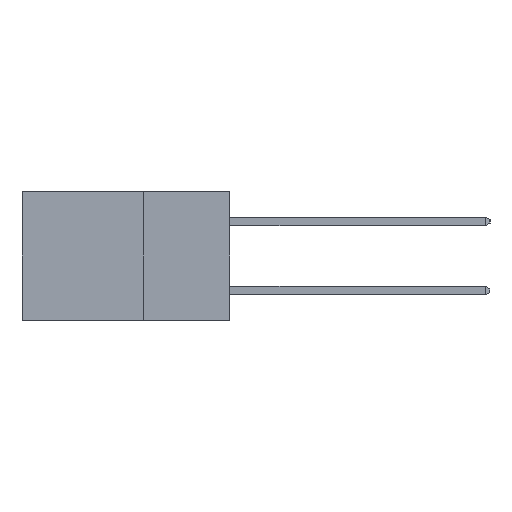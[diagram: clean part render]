
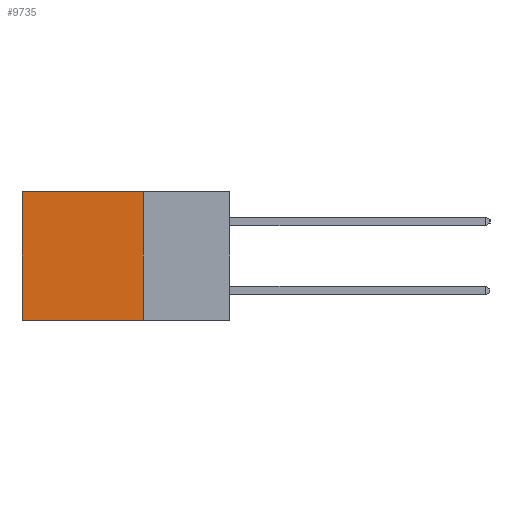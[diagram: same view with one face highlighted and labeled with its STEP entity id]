
A CAD part, left-side view. The second image highlights one B-rep face of the part: STEP entity #9735.
In plain terms, the highlighted planar face has unit normal (-1, 0, 0).
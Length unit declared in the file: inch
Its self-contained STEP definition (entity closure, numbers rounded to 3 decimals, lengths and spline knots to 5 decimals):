
#95 = CARTESIAN_POINT ( 'NONE',  ( 0.298, 0.25, 0. ) ) ;
#1175 = VERTEX_POINT ( 'NONE', #10415 ) ;
#1564 = VERTEX_POINT ( 'NONE', #8498 ) ;
#1645 = DIRECTION ( 'NONE',  ( 0., 1., 0. ) ) ;
#1934 = EDGE_LOOP ( 'NONE', ( #9062, #13494, #11848, #5618 ) ) ;
#1949 = VERTEX_POINT ( 'NONE', #3498 ) ;
#2283 = LINE ( 'NONE', #4247, #5204 ) ;
#2879 = LINE ( 'NONE', #8456, #8440 ) ;
#3411 = LINE ( 'NONE', #8245, #8972 ) ;
#3498 = CARTESIAN_POINT ( 'NONE',  ( 0.298, 0.6, 0. ) ) ;
#3585 = EDGE_CURVE ( 'NONE', #1564, #1949, #2283, .T. ) ;
#4247 = CARTESIAN_POINT ( 'NONE',  ( 0.298, 0.25, 0. ) ) ;
#4409 = FACE_OUTER_BOUND ( 'NONE', #1934, .T. ) ;
#4459 = VERTEX_POINT ( 'NONE', #10061 ) ;
#5204 = VECTOR ( 'NONE', #10838, 39.37008 ) ;
#5450 = VECTOR ( 'NONE', #1645, 39.37008 ) ;
#5618 = ORIENTED_EDGE ( 'NONE', *, *, #3585, .T. ) ;
#5648 = DIRECTION ( 'NONE',  ( 1., 0., 0. ) ) ;
#8245 = CARTESIAN_POINT ( 'NONE',  ( 0.298, 0.6, 0. ) ) ;
#8440 = VECTOR ( 'NONE', #11726, 39.37008 ) ;
#8456 = CARTESIAN_POINT ( 'NONE',  ( 0.298, 0.25, 0. ) ) ;
#8498 = CARTESIAN_POINT ( 'NONE',  ( 0.298, 0.25, 0. ) ) ;
#8774 = LINE ( 'NONE', #13726, #5450 ) ;
#8972 = VECTOR ( 'NONE', #10403, 39.37008 ) ;
#9062 = ORIENTED_EDGE ( 'NONE', *, *, #12751, .T. ) ;
#9312 = EDGE_CURVE ( 'NONE', #1175, #4459, #8774, .T. ) ;
#9735 = ADVANCED_FACE ( 'NONE', ( #4409 ), #10084, .F. ) ;
#10061 = CARTESIAN_POINT ( 'NONE',  ( 0.298, 0.6, -0.37 ) ) ;
#10084 = PLANE ( 'NONE',  #11988 ) ;
#10403 = DIRECTION ( 'NONE',  ( 0., 0., -1. ) ) ;
#10415 = CARTESIAN_POINT ( 'NONE',  ( 0.298, 0.25, -0.37 ) ) ;
#10838 = DIRECTION ( 'NONE',  ( 0., 1., 0. ) ) ;
#11726 = DIRECTION ( 'NONE',  ( 0., 0., -1. ) ) ;
#11848 = ORIENTED_EDGE ( 'NONE', *, *, #14084, .F. ) ;
#11988 = AXIS2_PLACEMENT_3D ( 'NONE', #95, #5648, #12266 ) ;
#12266 = DIRECTION ( 'NONE',  ( 0., 0., -1. ) ) ;
#12751 = EDGE_CURVE ( 'NONE', #1949, #4459, #3411, .T. ) ;
#13494 = ORIENTED_EDGE ( 'NONE', *, *, #9312, .F. ) ;
#13726 = CARTESIAN_POINT ( 'NONE',  ( 0.298, 0.25, -0.37 ) ) ;
#14084 = EDGE_CURVE ( 'NONE', #1564, #1175, #2879, .T. ) ;
